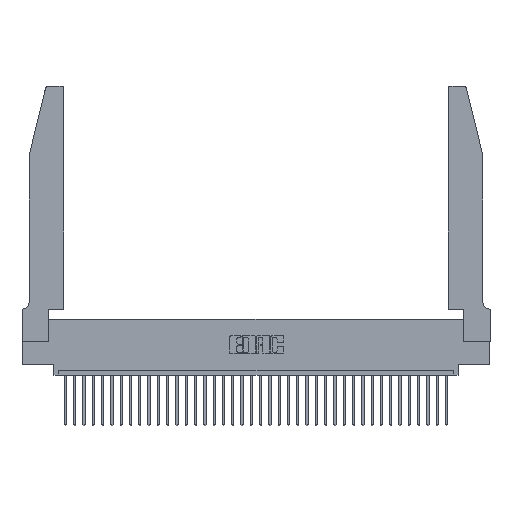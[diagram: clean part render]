
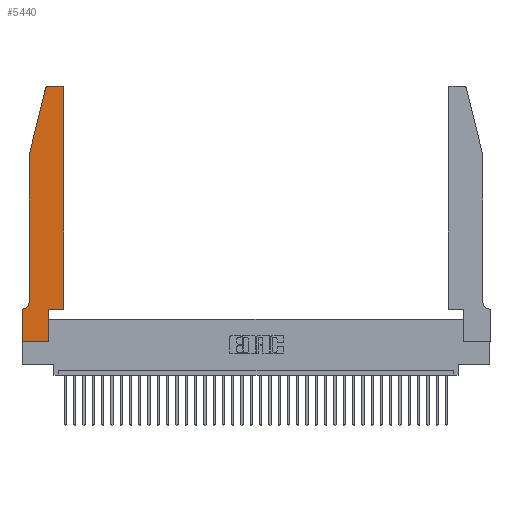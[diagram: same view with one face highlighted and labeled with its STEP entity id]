
A CAD part, top view. The second image highlights one B-rep face of the part: STEP entity #5440.
In plain terms, the highlighted planar face has unit normal (0, 0, 1).
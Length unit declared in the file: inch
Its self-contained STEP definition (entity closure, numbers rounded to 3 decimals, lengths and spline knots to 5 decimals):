
#283 = VERTEX_POINT ( 'NONE', #7094 ) ;
#349 = CARTESIAN_POINT ( 'NONE',  ( 0.25487, 2.72718, 0.37 ) ) ;
#1543 = CARTESIAN_POINT ( 'NONE',  ( 0.284, 2.72, 0.37 ) ) ;
#1733 = CARTESIAN_POINT ( 'NONE',  ( 0.0755, 2., 0.37 ) ) ;
#2132 = EDGE_CURVE ( 'NONE', #15163, #33766, #28618, .T. ) ;
#2236 = EDGE_CURVE ( 'NONE', #33790, #15163, #27300, .T. ) ;
#2651 = EDGE_LOOP ( 'NONE', ( #12482, #21282, #19412, #17972, #4943, #19094, #27359, #27757, #8569, #9618, #5339, #19651 ) ) ;
#2857 = VECTOR ( 'NONE', #25820, 39.37008 ) ;
#3547 = CARTESIAN_POINT ( 'NONE',  ( 0.0755, 2., 0.37 ) ) ;
#3787 = VERTEX_POINT ( 'NONE', #25446 ) ;
#4523 = VECTOR ( 'NONE', #27350, 39.37008 ) ;
#4943 = ORIENTED_EDGE ( 'NONE', *, *, #31176, .T. ) ;
#5339 = ORIENTED_EDGE ( 'NONE', *, *, #34037, .T. ) ;
#5440 = ADVANCED_FACE ( 'NONE', ( #27535 ), #21729, .T. ) ;
#6551 = VECTOR ( 'NONE', #33462, 39.37008 ) ;
#6632 = DIRECTION ( 'NONE',  ( -1., 0., 0. ) ) ;
#6786 = DIRECTION ( 'NONE',  ( 0., 0., 1. ) ) ;
#6826 = LINE ( 'NONE', #24861, #2857 ) ;
#7094 = CARTESIAN_POINT ( 'NONE',  ( 0.2865, 0.35, 0.37 ) ) ;
#7226 = CARTESIAN_POINT ( 'NONE',  ( 0.4205, 2.75, 0.37 ) ) ;
#7431 = CARTESIAN_POINT ( 'NONE',  ( 0.4505, 0.35, 0.37 ) ) ;
#8067 = VECTOR ( 'NONE', #35443, 39.37008 ) ;
#8206 = LINE ( 'NONE', #19559, #19641 ) ;
#8569 = ORIENTED_EDGE ( 'NONE', *, *, #9757, .T. ) ;
#9336 = LINE ( 'NONE', #15703, #8067 ) ;
#9618 = ORIENTED_EDGE ( 'NONE', *, *, #35353, .T. ) ;
#9733 = DIRECTION ( 'NONE',  ( 1., 0., 0. ) ) ;
#9757 = EDGE_CURVE ( 'NONE', #32794, #283, #31721, .T. ) ;
#9856 = CARTESIAN_POINT ( 'NONE',  ( 0.4205, 2.72, 0.37 ) ) ;
#10303 = AXIS2_PLACEMENT_3D ( 'NONE', #19152, #27569, #10651 ) ;
#10651 = DIRECTION ( 'NONE',  ( 1., 0., 0. ) ) ;
#10928 = EDGE_CURVE ( 'NONE', #3787, #33790, #31695, .T. ) ;
#11345 = VERTEX_POINT ( 'NONE', #7226 ) ;
#12175 = EDGE_CURVE ( 'NONE', #15457, #32794, #8206, .T. ) ;
#12482 = ORIENTED_EDGE ( 'NONE', *, *, #23610, .T. ) ;
#12764 = EDGE_CURVE ( 'NONE', #13475, #15457, #6826, .T. ) ;
#12947 = DIRECTION ( 'NONE',  ( 0., 1., 0. ) ) ;
#13475 = VERTEX_POINT ( 'NONE', #27340 ) ;
#13488 = AXIS2_PLACEMENT_3D ( 'NONE', #9856, #6786, #9733 ) ;
#13678 = VECTOR ( 'NONE', #36050, 39.37008 ) ;
#14618 = DIRECTION ( 'NONE',  ( -0.239, -0.971, 0. ) ) ;
#15163 = VERTEX_POINT ( 'NONE', #1733 ) ;
#15457 = VERTEX_POINT ( 'NONE', #19916 ) ;
#15703 = CARTESIAN_POINT ( 'NONE',  ( 0.4505, 0.35, 0.37 ) ) ;
#16557 = AXIS2_PLACEMENT_3D ( 'NONE', #26007, #20300, #29109 ) ;
#17730 = AXIS2_PLACEMENT_3D ( 'NONE', #1543, #18547, #26581 ) ;
#17972 = ORIENTED_EDGE ( 'NONE', *, *, #2132, .T. ) ;
#18385 = CIRCLE ( 'NONE', #13488, 0.03 ) ;
#18547 = DIRECTION ( 'NONE',  ( 0., 0., 1. ) ) ;
#18617 = LINE ( 'NONE', #24005, #4523 ) ;
#19094 = ORIENTED_EDGE ( 'NONE', *, *, #21393, .T. ) ;
#19152 = CARTESIAN_POINT ( 'NONE',  ( 0., 0.35, 0.37 ) ) ;
#19412 = ORIENTED_EDGE ( 'NONE', *, *, #2236, .T. ) ;
#19559 = CARTESIAN_POINT ( 'NONE',  ( 0., 0., 0.37 ) ) ;
#19641 = VECTOR ( 'NONE', #30803, 39.37008 ) ;
#19651 = ORIENTED_EDGE ( 'NONE', *, *, #31395, .T. ) ;
#19916 = CARTESIAN_POINT ( 'NONE',  ( 0., 0., 0.37 ) ) ;
#20190 = VECTOR ( 'NONE', #14618, 39.37008 ) ;
#20300 = DIRECTION ( 'NONE',  ( 0., 0., -1. ) ) ;
#21282 = ORIENTED_EDGE ( 'NONE', *, *, #10928, .T. ) ;
#21393 = EDGE_CURVE ( 'NONE', #31367, #13475, #18617, .T. ) ;
#21729 = PLANE ( 'NONE',  #10303 ) ;
#22998 = VECTOR ( 'NONE', #12947, 39.37008 ) ;
#23610 = EDGE_CURVE ( 'NONE', #11345, #3787, #33010, .T. ) ;
#23743 = CARTESIAN_POINT ( 'NONE',  ( 0.2605, 2.75, 0.37 ) ) ;
#23943 = LINE ( 'NONE', #7431, #22998 ) ;
#24005 = CARTESIAN_POINT ( 'NONE',  ( 0.0755, 0.35, 0.37 ) ) ;
#24738 = VERTEX_POINT ( 'NONE', #27907 ) ;
#24861 = CARTESIAN_POINT ( 'NONE',  ( 0., 0., 0.37 ) ) ;
#25446 = CARTESIAN_POINT ( 'NONE',  ( 0.284, 2.75, 0.37 ) ) ;
#25820 = DIRECTION ( 'NONE',  ( 0., -1., 0. ) ) ;
#26007 = CARTESIAN_POINT ( 'NONE',  ( 0.0055, 0.42, 0.37 ) ) ;
#26581 = DIRECTION ( 'NONE',  ( 1., 0., 0. ) ) ;
#26756 = CARTESIAN_POINT ( 'NONE',  ( 0.0055, 0.35, 0.37 ) ) ;
#26768 = VERTEX_POINT ( 'NONE', #36423 ) ;
#27300 = LINE ( 'NONE', #3547, #20190 ) ;
#27340 = CARTESIAN_POINT ( 'NONE',  ( 0., 0.35, 0.37 ) ) ;
#27350 = DIRECTION ( 'NONE',  ( -1., 0., 0. ) ) ;
#27359 = ORIENTED_EDGE ( 'NONE', *, *, #12764, .T. ) ;
#27535 = FACE_OUTER_BOUND ( 'NONE', #2651, .T. ) ;
#27569 = DIRECTION ( 'NONE',  ( 0., 0., 1. ) ) ;
#27657 = CARTESIAN_POINT ( 'NONE',  ( 0.2865, 0., 0.37 ) ) ;
#27757 = ORIENTED_EDGE ( 'NONE', *, *, #12175, .T. ) ;
#27907 = CARTESIAN_POINT ( 'NONE',  ( 0.4505, 0.35, 0.37 ) ) ;
#28618 = LINE ( 'NONE', #32629, #6551 ) ;
#29109 = DIRECTION ( 'NONE',  ( -1., 0., 0. ) ) ;
#30275 = CARTESIAN_POINT ( 'NONE',  ( 0.2865, 0.35, 0.37 ) ) ;
#30803 = DIRECTION ( 'NONE',  ( 1., 0., 0. ) ) ;
#31176 = EDGE_CURVE ( 'NONE', #33766, #31367, #32994, .T. ) ;
#31319 = CARTESIAN_POINT ( 'NONE',  ( 0.0755, 0.42, 0.37 ) ) ;
#31367 = VERTEX_POINT ( 'NONE', #26756 ) ;
#31395 = EDGE_CURVE ( 'NONE', #26768, #11345, #18385, .T. ) ;
#31695 = CIRCLE ( 'NONE', #17730, 0.03 ) ;
#31721 = LINE ( 'NONE', #30275, #13678 ) ;
#32629 = CARTESIAN_POINT ( 'NONE',  ( 0.0755, 2., 0.37 ) ) ;
#32794 = VERTEX_POINT ( 'NONE', #27657 ) ;
#32994 = CIRCLE ( 'NONE', #16557, 0.07 ) ;
#33010 = LINE ( 'NONE', #23743, #33869 ) ;
#33462 = DIRECTION ( 'NONE',  ( 0., -1., 0. ) ) ;
#33766 = VERTEX_POINT ( 'NONE', #31319 ) ;
#33790 = VERTEX_POINT ( 'NONE', #349 ) ;
#33869 = VECTOR ( 'NONE', #6632, 39.37008 ) ;
#34037 = EDGE_CURVE ( 'NONE', #24738, #26768, #23943, .T. ) ;
#35353 = EDGE_CURVE ( 'NONE', #283, #24738, #9336, .T. ) ;
#35443 = DIRECTION ( 'NONE',  ( 1., 0., 0. ) ) ;
#36050 = DIRECTION ( 'NONE',  ( 0., 1., 0. ) ) ;
#36423 = CARTESIAN_POINT ( 'NONE',  ( 0.4505, 2.72, 0.37 ) ) ;
